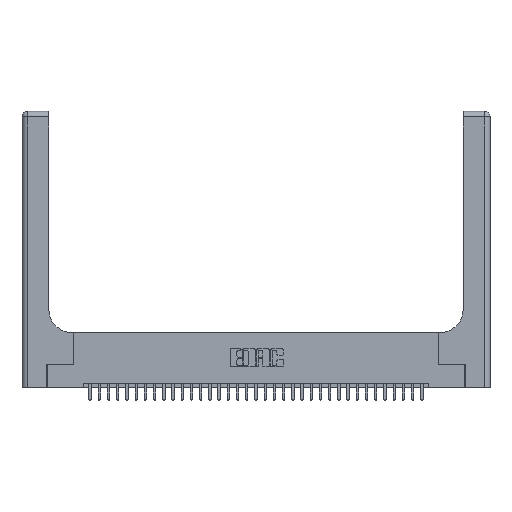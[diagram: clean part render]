
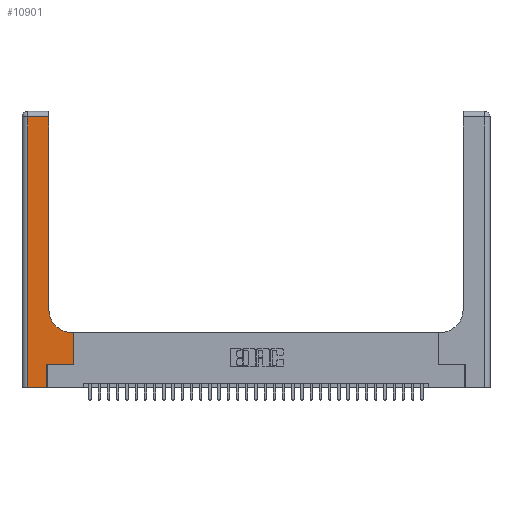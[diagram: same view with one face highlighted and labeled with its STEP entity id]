
A CAD part, top view. The second image highlights one B-rep face of the part: STEP entity #10901.
In plain terms, the highlighted planar face has unit normal (0, 0, 1).
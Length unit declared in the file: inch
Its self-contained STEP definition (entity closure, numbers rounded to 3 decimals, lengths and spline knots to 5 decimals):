
#559 = CARTESIAN_POINT ( 'NONE',  ( 0., 2.94, 0.37 ) ) ;
#1154 = ORIENTED_EDGE ( 'NONE', *, *, #5722, .T. ) ;
#1215 = CARTESIAN_POINT ( 'NONE',  ( 0.2915, 2.94, 0.37 ) ) ;
#1964 = CARTESIAN_POINT ( 'NONE',  ( 0.269, 0., 0.37 ) ) ;
#2220 = CARTESIAN_POINT ( 'NONE',  ( 0.269, 0., 0.37 ) ) ;
#2958 = DIRECTION ( 'NONE',  ( 0., 0., -1. ) ) ;
#3439 = CARTESIAN_POINT ( 'NONE',  ( 0.5415, 0.85, 0.37 ) ) ;
#5028 = EDGE_CURVE ( 'NONE', #28687, #7713, #12130, .T. ) ;
#5383 = PLANE ( 'NONE',  #19724 ) ;
#5722 = EDGE_CURVE ( 'NONE', #29704, #16946, #11672, .T. ) ;
#5907 = VERTEX_POINT ( 'NONE', #27442 ) ;
#5965 = CARTESIAN_POINT ( 'NONE',  ( 0.2915, 0.6, 0.37 ) ) ;
#6184 = ORIENTED_EDGE ( 'NONE', *, *, #5028, .T. ) ;
#6194 = DIRECTION ( 'NONE',  ( 1., 0., 0. ) ) ;
#6216 = VERTEX_POINT ( 'NONE', #26569 ) ;
#7141 = CARTESIAN_POINT ( 'NONE',  ( 0.5585, 0.25, 0.37 ) ) ;
#7713 = VERTEX_POINT ( 'NONE', #17292 ) ;
#9828 = DIRECTION ( 'NONE',  ( 0., 1., 0. ) ) ;
#9939 = DIRECTION ( 'NONE',  ( 1., 0., 0. ) ) ;
#10223 = CARTESIAN_POINT ( 'NONE',  ( 0.06, 2.94, 0.37 ) ) ;
#10629 = VERTEX_POINT ( 'NONE', #15151 ) ;
#10901 = ADVANCED_FACE ( 'NONE', ( #18307 ), #5383, .F. ) ;
#11672 = LINE ( 'NONE', #26738, #25163 ) ;
#12130 = LINE ( 'NONE', #2220, #18465 ) ;
#12520 = CARTESIAN_POINT ( 'NONE',  ( 0.2915, 0.85, 0.37 ) ) ;
#12937 = VECTOR ( 'NONE', #16826, 39.37008 ) ;
#13163 = DIRECTION ( 'NONE',  ( 0., 1., 0. ) ) ;
#13264 = CARTESIAN_POINT ( 'NONE',  ( 0., 0., 0.37 ) ) ;
#13314 = LINE ( 'NONE', #559, #19651 ) ;
#14090 = CARTESIAN_POINT ( 'NONE',  ( 0.06, 3., 0.37 ) ) ;
#14161 = CIRCLE ( 'NONE', #31870, 0.25 ) ;
#15151 = CARTESIAN_POINT ( 'NONE',  ( 0.5585, 0.6, 0.37 ) ) ;
#16216 = CARTESIAN_POINT ( 'NONE',  ( 0., 3., 0.37 ) ) ;
#16385 = ORIENTED_EDGE ( 'NONE', *, *, #25004, .T. ) ;
#16668 = DIRECTION ( 'NONE',  ( -1., 0., 0. ) ) ;
#16826 = DIRECTION ( 'NONE',  ( 0., -1., 0. ) ) ;
#16898 = DIRECTION ( 'NONE',  ( -1., 0., 0. ) ) ;
#16946 = VERTEX_POINT ( 'NONE', #1215 ) ;
#17259 = ORIENTED_EDGE ( 'NONE', *, *, #21953, .T. ) ;
#17292 = CARTESIAN_POINT ( 'NONE',  ( 0.269, 0.25, 0.37 ) ) ;
#18039 = EDGE_CURVE ( 'NONE', #10629, #6216, #20098, .T. ) ;
#18307 = FACE_OUTER_BOUND ( 'NONE', #31361, .T. ) ;
#18465 = VECTOR ( 'NONE', #26428, 39.37008 ) ;
#18629 = CARTESIAN_POINT ( 'NONE',  ( 0.5585, 0.25, 0.37 ) ) ;
#18917 = DIRECTION ( 'NONE',  ( -1., 0., 0. ) ) ;
#19651 = VECTOR ( 'NONE', #16898, 39.37008 ) ;
#19724 = AXIS2_PLACEMENT_3D ( 'NONE', #16216, #2958, #18917 ) ;
#20098 = LINE ( 'NONE', #5965, #26427 ) ;
#20331 = LINE ( 'NONE', #13264, #33774 ) ;
#21265 = EDGE_CURVE ( 'NONE', #22842, #5907, #27295, .T. ) ;
#21952 = EDGE_CURVE ( 'NONE', #6216, #29704, #14161, .T. ) ;
#21953 = EDGE_CURVE ( 'NONE', #16946, #22842, #13314, .T. ) ;
#22315 = DIRECTION ( 'NONE',  ( 0., 0., -1. ) ) ;
#22842 = VERTEX_POINT ( 'NONE', #10223 ) ;
#23395 = ORIENTED_EDGE ( 'NONE', *, *, #18039, .T. ) ;
#23659 = EDGE_CURVE ( 'NONE', #24317, #10629, #26282, .T. ) ;
#23686 = EDGE_CURVE ( 'NONE', #7713, #24317, #32565, .T. ) ;
#24317 = VERTEX_POINT ( 'NONE', #18629 ) ;
#24403 = ORIENTED_EDGE ( 'NONE', *, *, #23659, .T. ) ;
#24600 = VECTOR ( 'NONE', #9939, 39.37008 ) ;
#25004 = EDGE_CURVE ( 'NONE', #5907, #28687, #20331, .T. ) ;
#25163 = VECTOR ( 'NONE', #13163, 39.37008 ) ;
#25638 = ORIENTED_EDGE ( 'NONE', *, *, #21265, .T. ) ;
#25777 = ORIENTED_EDGE ( 'NONE', *, *, #21952, .T. ) ;
#26100 = CARTESIAN_POINT ( 'NONE',  ( 0.269, 0.25, 0.37 ) ) ;
#26282 = LINE ( 'NONE', #7141, #33402 ) ;
#26427 = VECTOR ( 'NONE', #16668, 39.37008 ) ;
#26428 = DIRECTION ( 'NONE',  ( 0., 1., 0. ) ) ;
#26569 = CARTESIAN_POINT ( 'NONE',  ( 0.5415, 0.6, 0.37 ) ) ;
#26738 = CARTESIAN_POINT ( 'NONE',  ( 0.2915, 3., 0.37 ) ) ;
#27295 = LINE ( 'NONE', #14090, #12937 ) ;
#27361 = ORIENTED_EDGE ( 'NONE', *, *, #23686, .T. ) ;
#27442 = CARTESIAN_POINT ( 'NONE',  ( 0.06, 0., 0.37 ) ) ;
#28687 = VERTEX_POINT ( 'NONE', #1964 ) ;
#29415 = DIRECTION ( 'NONE',  ( 1., 0., 0. ) ) ;
#29704 = VERTEX_POINT ( 'NONE', #12520 ) ;
#31361 = EDGE_LOOP ( 'NONE', ( #1154, #17259, #25638, #16385, #6184, #27361, #24403, #23395, #25777 ) ) ;
#31870 = AXIS2_PLACEMENT_3D ( 'NONE', #3439, #22315, #6194 ) ;
#32565 = LINE ( 'NONE', #26100, #24600 ) ;
#33402 = VECTOR ( 'NONE', #9828, 39.37008 ) ;
#33774 = VECTOR ( 'NONE', #29415, 39.37008 ) ;
